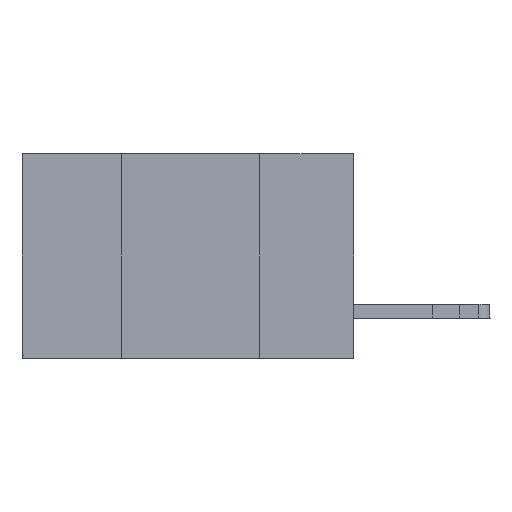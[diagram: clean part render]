
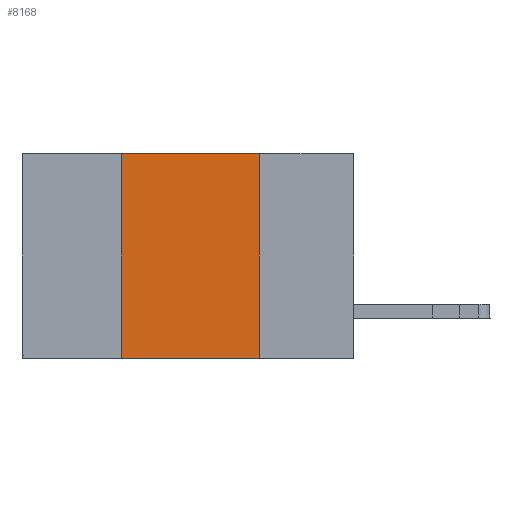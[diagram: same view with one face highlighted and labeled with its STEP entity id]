
A CAD part, left-side view. The second image highlights one B-rep face of the part: STEP entity #8168.
In plain terms, the highlighted planar face has unit normal (-1, 0, 0).
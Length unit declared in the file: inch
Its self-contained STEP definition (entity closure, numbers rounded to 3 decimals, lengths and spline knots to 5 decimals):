
#699 = LINE ( 'NONE', #13148, #10712 ) ;
#1066 = CARTESIAN_POINT ( 'NONE',  ( 0., 0.42, -0.37 ) ) ;
#1150 = ORIENTED_EDGE ( 'NONE', *, *, #11738, .F. ) ;
#1187 = DIRECTION ( 'NONE',  ( 0., -1., 0. ) ) ;
#1588 = EDGE_CURVE ( 'NONE', #12494, #11898, #8241, .T. ) ;
#1630 = CARTESIAN_POINT ( 'NONE',  ( 0., 0.17, 0. ) ) ;
#2545 = CARTESIAN_POINT ( 'NONE',  ( 0., 0.17, -0.37 ) ) ;
#2640 = ORIENTED_EDGE ( 'NONE', *, *, #1588, .F. ) ;
#3382 = LINE ( 'NONE', #9282, #13772 ) ;
#3549 = VECTOR ( 'NONE', #7263, 39.37008 ) ;
#3745 = CARTESIAN_POINT ( 'NONE',  ( 0., 0.6, 0. ) ) ;
#3977 = LINE ( 'NONE', #1630, #3549 ) ;
#5084 = EDGE_CURVE ( 'NONE', #13818, #10866, #3382, .T. ) ;
#6582 = PLANE ( 'NONE',  #16623 ) ;
#7263 = DIRECTION ( 'NONE',  ( 0., 0., -1. ) ) ;
#7893 = DIRECTION ( 'NONE',  ( 0., 0., -1. ) ) ;
#8135 = DIRECTION ( 'NONE',  ( 0., 0., 1. ) ) ;
#8168 = ADVANCED_FACE ( 'NONE', ( #15352 ), #6582, .F. ) ;
#8241 = LINE ( 'NONE', #14230, #16430 ) ;
#8485 = EDGE_LOOP ( 'NONE', ( #1150, #2640, #12559, #11458 ) ) ;
#9282 = CARTESIAN_POINT ( 'NONE',  ( 0., 0.6, -0.37 ) ) ;
#10159 = CARTESIAN_POINT ( 'NONE',  ( 0., 0.17, 0. ) ) ;
#10712 = VECTOR ( 'NONE', #8135, 39.37008 ) ;
#10866 = VERTEX_POINT ( 'NONE', #2545 ) ;
#11458 = ORIENTED_EDGE ( 'NONE', *, *, #5084, .T. ) ;
#11531 = EDGE_CURVE ( 'NONE', #13818, #12494, #699, .T. ) ;
#11738 = EDGE_CURVE ( 'NONE', #11898, #10866, #3977, .T. ) ;
#11898 = VERTEX_POINT ( 'NONE', #10159 ) ;
#12494 = VERTEX_POINT ( 'NONE', #14877 ) ;
#12559 = ORIENTED_EDGE ( 'NONE', *, *, #11531, .F. ) ;
#13148 = CARTESIAN_POINT ( 'NONE',  ( 0., 0.42, 0. ) ) ;
#13772 = VECTOR ( 'NONE', #1187, 39.37008 ) ;
#13818 = VERTEX_POINT ( 'NONE', #1066 ) ;
#14094 = DIRECTION ( 'NONE',  ( 0., -1., 0. ) ) ;
#14230 = CARTESIAN_POINT ( 'NONE',  ( 0., 0.6, 0. ) ) ;
#14877 = CARTESIAN_POINT ( 'NONE',  ( 0., 0.42, 0. ) ) ;
#15309 = DIRECTION ( 'NONE',  ( 1., 0., 0. ) ) ;
#15352 = FACE_OUTER_BOUND ( 'NONE', #8485, .T. ) ;
#16430 = VECTOR ( 'NONE', #14094, 39.37008 ) ;
#16623 = AXIS2_PLACEMENT_3D ( 'NONE', #3745, #15309, #7893 ) ;
